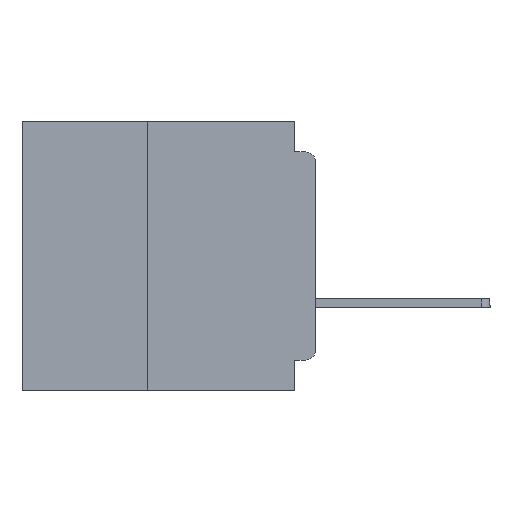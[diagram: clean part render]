
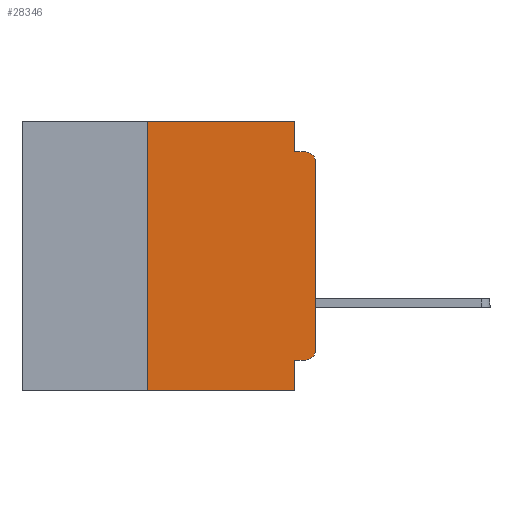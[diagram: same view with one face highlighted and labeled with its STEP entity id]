
A CAD part, left-side view. The second image highlights one B-rep face of the part: STEP entity #28346.
In plain terms, the highlighted planar face has unit normal (-1, 0, 0).
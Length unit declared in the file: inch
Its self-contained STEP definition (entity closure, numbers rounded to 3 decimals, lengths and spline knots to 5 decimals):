
#2508 = CARTESIAN_POINT ( 'NONE',  ( 0., 0., -0.06 ) ) ;
#3865 = VERTEX_POINT ( 'NONE', #13871 ) ;
#4545 = DIRECTION ( 'NONE',  ( 0., 0., -1. ) ) ;
#4812 = PLANE ( 'NONE',  #49418 ) ;
#5232 = VECTOR ( 'NONE', #51412, 39.37008 ) ;
#5716 = CARTESIAN_POINT ( 'NONE',  ( 0., 0.25, -0.4 ) ) ;
#6724 = CARTESIAN_POINT ( 'NONE',  ( 0., 0.25, 0. ) ) ;
#9420 = CARTESIAN_POINT ( 'NONE',  ( 0., 0.015, -0.045 ) ) ;
#10131 = LINE ( 'NONE', #34694, #44414 ) ;
#10438 = LINE ( 'NONE', #28395, #31974 ) ;
#10552 = LINE ( 'NONE', #16744, #20653 ) ;
#10766 = ORIENTED_EDGE ( 'NONE', *, *, #50670, .F. ) ;
#10839 = DIRECTION ( 'NONE',  ( 0., -1., 0. ) ) ;
#10840 = DIRECTION ( 'NONE',  ( -1., 0., 0. ) ) ;
#11653 = CARTESIAN_POINT ( 'NONE',  ( 0., 0.25, -0.4 ) ) ;
#12025 = CARTESIAN_POINT ( 'NONE',  ( 0., 0.031, -0.045 ) ) ;
#12106 = CIRCLE ( 'NONE', #27533, 0.015 ) ;
#12406 = DIRECTION ( 'NONE',  ( 0., -1., 0. ) ) ;
#12731 = LINE ( 'NONE', #11653, #22790 ) ;
#13358 = VERTEX_POINT ( 'NONE', #18582 ) ;
#13552 = DIRECTION ( 'NONE',  ( 1., 0., 0. ) ) ;
#13871 = CARTESIAN_POINT ( 'NONE',  ( 0., 0.015, -0.355 ) ) ;
#14139 = DIRECTION ( 'NONE',  ( -1., 0., 0. ) ) ;
#14530 = AXIS2_PLACEMENT_3D ( 'NONE', #36577, #10840, #40882 ) ;
#14813 = ORIENTED_EDGE ( 'NONE', *, *, #41432, .T. ) ;
#16744 = CARTESIAN_POINT ( 'NONE',  ( 0., 0., -0.045 ) ) ;
#16752 = CIRCLE ( 'NONE', #14530, 0.015 ) ;
#18582 = CARTESIAN_POINT ( 'NONE',  ( 0., 0., -0.34 ) ) ;
#18829 = VERTEX_POINT ( 'NONE', #18932 ) ;
#18932 = CARTESIAN_POINT ( 'NONE',  ( 0., 0.031, -0.355 ) ) ;
#19944 = DIRECTION ( 'NONE',  ( 0., 0., 1. ) ) ;
#20274 = ORIENTED_EDGE ( 'NONE', *, *, #50996, .T. ) ;
#20653 = VECTOR ( 'NONE', #12406, 39.37008 ) ;
#20719 = FACE_OUTER_BOUND ( 'NONE', #50202, .T. ) ;
#20754 = VECTOR ( 'NONE', #10839, 39.37008 ) ;
#21636 = VERTEX_POINT ( 'NONE', #55530 ) ;
#22790 = VECTOR ( 'NONE', #46020, 39.37008 ) ;
#23547 = EDGE_CURVE ( 'NONE', #3865, #18829, #51043, .T. ) ;
#23784 = ORIENTED_EDGE ( 'NONE', *, *, #37240, .F. ) ;
#23838 = DIRECTION ( 'NONE',  ( 0., -1., 0. ) ) ;
#24034 = DIRECTION ( 'NONE',  ( 0., 0., -1. ) ) ;
#24553 = VERTEX_POINT ( 'NONE', #6724 ) ;
#24766 = EDGE_CURVE ( 'NONE', #28764, #53794, #10552, .T. ) ;
#27533 = AXIS2_PLACEMENT_3D ( 'NONE', #39847, #14139, #44166 ) ;
#27716 = VERTEX_POINT ( 'NONE', #5716 ) ;
#27865 = EDGE_CURVE ( 'NONE', #21636, #28764, #37557, .T. ) ;
#28346 = ADVANCED_FACE ( 'NONE', ( #20719 ), #4812, .F. ) ;
#28395 = CARTESIAN_POINT ( 'NONE',  ( 0., 0., 0. ) ) ;
#28764 = VERTEX_POINT ( 'NONE', #12025 ) ;
#29935 = ORIENTED_EDGE ( 'NONE', *, *, #39313, .F. ) ;
#30371 = ORIENTED_EDGE ( 'NONE', *, *, #27865, .F. ) ;
#31974 = VECTOR ( 'NONE', #19944, 39.37008 ) ;
#34694 = CARTESIAN_POINT ( 'NONE',  ( 0., 0.031, -0.4 ) ) ;
#34828 = LINE ( 'NONE', #40694, #20754 ) ;
#36213 = VECTOR ( 'NONE', #24034, 39.37008 ) ;
#36577 = CARTESIAN_POINT ( 'NONE',  ( 0., 0.015, -0.34 ) ) ;
#37240 = EDGE_CURVE ( 'NONE', #18829, #53384, #10131, .T. ) ;
#37557 = LINE ( 'NONE', #45420, #36213 ) ;
#39255 = CARTESIAN_POINT ( 'NONE',  ( 0., 0.437, 0. ) ) ;
#39313 = EDGE_CURVE ( 'NONE', #24553, #21636, #34828, .T. ) ;
#39847 = CARTESIAN_POINT ( 'NONE',  ( 0., 0.015, -0.06 ) ) ;
#40615 = VECTOR ( 'NONE', #23838, 39.37008 ) ;
#40694 = CARTESIAN_POINT ( 'NONE',  ( 0., 0.437, 0. ) ) ;
#40882 = DIRECTION ( 'NONE',  ( 0., 0., -1. ) ) ;
#40936 = VERTEX_POINT ( 'NONE', #2508 ) ;
#40970 = EDGE_CURVE ( 'NONE', #13358, #40936, #10438, .T. ) ;
#41432 = EDGE_CURVE ( 'NONE', #27716, #53384, #41974, .T. ) ;
#41974 = LINE ( 'NONE', #45237, #40615 ) ;
#43577 = DIRECTION ( 'NONE',  ( 0., 0., -1. ) ) ;
#44166 = DIRECTION ( 'NONE',  ( 0., 0., -1. ) ) ;
#44414 = VECTOR ( 'NONE', #4545, 39.37008 ) ;
#45237 = CARTESIAN_POINT ( 'NONE',  ( 0., 0.437, -0.4 ) ) ;
#45420 = CARTESIAN_POINT ( 'NONE',  ( 0., 0.031, 0. ) ) ;
#46020 = DIRECTION ( 'NONE',  ( 0., 0., 1. ) ) ;
#47067 = CARTESIAN_POINT ( 'NONE',  ( 0., 0., -0.355 ) ) ;
#47871 = EDGE_CURVE ( 'NONE', #40936, #53794, #12106, .T. ) ;
#49072 = ORIENTED_EDGE ( 'NONE', *, *, #23547, .F. ) ;
#49418 = AXIS2_PLACEMENT_3D ( 'NONE', #39255, #13552, #43577 ) ;
#49723 = ORIENTED_EDGE ( 'NONE', *, *, #40970, .T. ) ;
#50202 = EDGE_LOOP ( 'NONE', ( #49723, #52146, #54250, #30371, #29935, #10766, #14813, #23784, #49072, #20274 ) ) ;
#50670 = EDGE_CURVE ( 'NONE', #27716, #24553, #12731, .T. ) ;
#50996 = EDGE_CURVE ( 'NONE', #3865, #13358, #16752, .T. ) ;
#51043 = LINE ( 'NONE', #47067, #5232 ) ;
#51412 = DIRECTION ( 'NONE',  ( 0., 1., 0. ) ) ;
#52146 = ORIENTED_EDGE ( 'NONE', *, *, #47871, .T. ) ;
#53384 = VERTEX_POINT ( 'NONE', #53457 ) ;
#53457 = CARTESIAN_POINT ( 'NONE',  ( 0., 0.031, -0.4 ) ) ;
#53794 = VERTEX_POINT ( 'NONE', #9420 ) ;
#54250 = ORIENTED_EDGE ( 'NONE', *, *, #24766, .F. ) ;
#55530 = CARTESIAN_POINT ( 'NONE',  ( 0., 0.031, 0. ) ) ;
